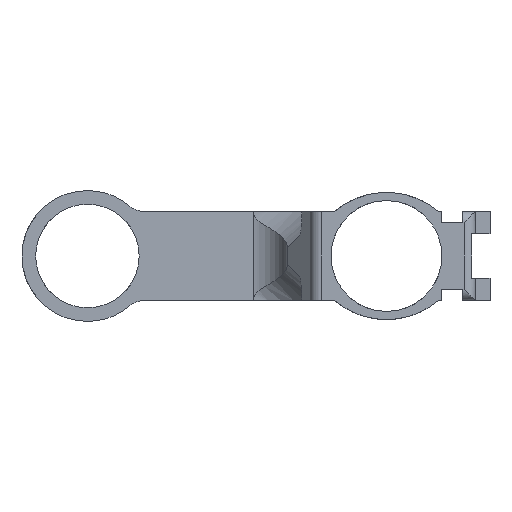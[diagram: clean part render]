
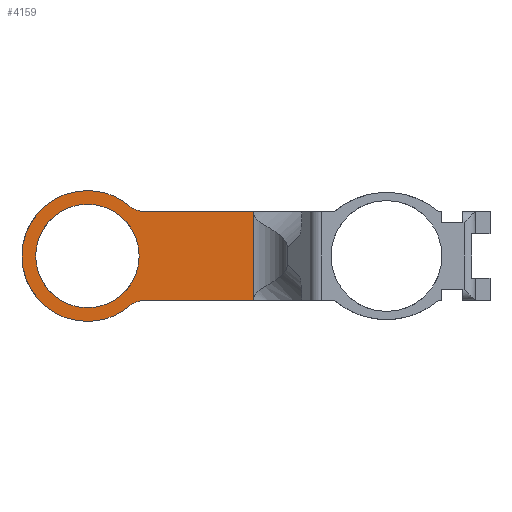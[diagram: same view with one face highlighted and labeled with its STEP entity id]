
A CAD part, left-side view. The second image highlights one B-rep face of the part: STEP entity #4159.
In plain terms, the highlighted planar face has unit normal (-1, 0, 0).
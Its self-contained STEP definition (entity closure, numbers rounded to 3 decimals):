
#380 = FACE_OUTER_BOUND ( 'NONE', #5228, .T. ) ;
#385 = FACE_BOUND ( 'NONE', #5230, .T. ) ;
#406 = CIRCLE ( 'NONE', #5538, 7. ) ;
#436 = CIRCLE ( 'NONE', #5544, 8.85 ) ;
#573 = LINE ( 'NONE', #3904, #576 ) ;
#576 = VECTOR ( 'NONE', #3905, 1000. ) ;
#577 = CIRCLE ( 'NONE', #3512, 8.85 ) ;
#1004 = CIRCLE ( 'NONE', #3519, 7. ) ;
#1006 = LINE ( 'NONE', #1348, #1010 ) ;
#1007 = LINE ( 'NONE', #1346, #1008 ) ;
#1008 = VECTOR ( 'NONE', #1347, 1000. ) ;
#1009 = CIRCLE ( 'NONE', #3520, 3. ) ;
#1010 = VECTOR ( 'NONE', #1349, 1000. ) ;
#1011 = CIRCLE ( 'NONE', #3521, 3. ) ;
#1012 = LINE ( 'NONE', #1350, #1014 ) ;
#1014 = VECTOR ( 'NONE', #1351, 1000. ) ;
#1143 = CIRCLE ( 'NONE', #3552, 8.85 ) ;
#1304 = CARTESIAN_POINT ( 'NONE',  ( -14., 40.45, 0. ) ) ;
#1305 = DIRECTION ( 'NONE',  ( -1., 0., 0. ) ) ;
#1306 = DIRECTION ( 'NONE',  ( 0., 1., 0. ) ) ;
#1346 = CARTESIAN_POINT ( 'NONE',  ( -14., 18.048, 6. ) ) ;
#1347 = DIRECTION ( 'NONE',  ( 0., 0., 1. ) ) ;
#1348 = CARTESIAN_POINT ( 'NONE',  ( -14., 18.024, 5.976 ) ) ;
#1349 = DIRECTION ( 'NONE',  ( 0., -0.707, 0.707 ) ) ;
#1350 = CARTESIAN_POINT ( 'NONE',  ( -14., 18.024, -5.976 ) ) ;
#1351 = DIRECTION ( 'NONE',  ( 0., 0.707, 0.707 ) ) ;
#1352 = CARTESIAN_POINT ( 'NONE',  ( -14., 32.741, 9. ) ) ;
#1353 = DIRECTION ( 'NONE',  ( 1., 0., 0. ) ) ;
#1354 = DIRECTION ( 'NONE',  ( 0., 1., 0. ) ) ;
#1355 = CARTESIAN_POINT ( 'NONE',  ( -14., 32.741, -9. ) ) ;
#1356 = DIRECTION ( 'NONE',  ( 1., 0., 0. ) ) ;
#1357 = DIRECTION ( 'NONE',  ( 0., 1., 0. ) ) ;
#1808 = CARTESIAN_POINT ( 'NONE',  ( -14., 40.45, 0. ) ) ;
#1809 = DIRECTION ( 'NONE',  ( -1., 0., 0. ) ) ;
#1810 = DIRECTION ( 'NONE',  ( 0., 1., 0. ) ) ;
#2225 = CARTESIAN_POINT ( 'NONE',  ( -14., 24.039, -6. ) ) ;
#2226 = DIRECTION ( 'NONE',  ( 0., -1., 0. ) ) ;
#2457 = LINE ( 'NONE', #2225, #2460 ) ;
#2460 = VECTOR ( 'NONE', #2226, 1000. ) ;
#2681 = CARTESIAN_POINT ( 'NONE',  ( -14., 49.3, -8.85 ) ) ;
#2686 = DIRECTION ( 'NONE',  ( 1., 0., 0. ) ) ;
#2688 = PLANE ( 'NONE',  #5525 ) ;
#2690 = DIRECTION ( 'NONE',  ( 0., 1., 0. ) ) ;
#2842 = CARTESIAN_POINT ( 'NONE',  ( -14., 40.45, 0. ) ) ;
#2843 = DIRECTION ( 'NONE',  ( -1., 0., 0. ) ) ;
#2844 = DIRECTION ( 'NONE',  ( 0., 1., 0. ) ) ;
#3123 = CARTESIAN_POINT ( 'NONE',  ( -14., 40.45, 0. ) ) ;
#3124 = DIRECTION ( 'NONE',  ( -1., 0., 0. ) ) ;
#3125 = DIRECTION ( 'NONE',  ( 0., 1., 0. ) ) ;
#3235 = CARTESIAN_POINT ( 'NONE',  ( -14., 34.693, -6.722 ) ) ;
#3236 = CARTESIAN_POINT ( 'NONE',  ( -14., 40.45, -7. ) ) ;
#3238 = CARTESIAN_POINT ( 'NONE',  ( -14., 40.45, 7. ) ) ;
#3260 = CARTESIAN_POINT ( 'NONE',  ( -14., 40.45, 8.85 ) ) ;
#3268 = CARTESIAN_POINT ( 'NONE',  ( -14., 40.45, -8.85 ) ) ;
#3290 = CARTESIAN_POINT ( 'NONE',  ( -14., 32.741, -6. ) ) ;
#3295 = CARTESIAN_POINT ( 'NONE',  ( -14., 18., -6. ) ) ;
#3388 = CARTESIAN_POINT ( 'NONE',  ( -14., 18., 6. ) ) ;
#3392 = CARTESIAN_POINT ( 'NONE',  ( -14., 32.741, 6. ) ) ;
#3394 = CARTESIAN_POINT ( 'NONE',  ( -14., 34.693, 6.722 ) ) ;
#3433 = CARTESIAN_POINT ( 'NONE',  ( -14., 18.048, 5.952 ) ) ;
#3435 = CARTESIAN_POINT ( 'NONE',  ( -14., 18.048, -5.952 ) ) ;
#3512 = AXIS2_PLACEMENT_3D ( 'NONE', #3916, #3917, #3918 ) ;
#3519 = AXIS2_PLACEMENT_3D ( 'NONE', #1304, #1305, #1306 ) ;
#3520 = AXIS2_PLACEMENT_3D ( 'NONE', #1352, #1353, #1354 ) ;
#3521 = AXIS2_PLACEMENT_3D ( 'NONE', #1355, #1356, #1357 ) ;
#3552 = AXIS2_PLACEMENT_3D ( 'NONE', #1808, #1809, #1810 ) ;
#3904 = CARTESIAN_POINT ( 'NONE',  ( -14., 12.842, 6. ) ) ;
#3905 = DIRECTION ( 'NONE',  ( 0., 1., 0. ) ) ;
#3916 = CARTESIAN_POINT ( 'NONE',  ( -14., 40.45, 0. ) ) ;
#3917 = DIRECTION ( 'NONE',  ( -1., 0., 0. ) ) ;
#3918 = DIRECTION ( 'NONE',  ( 0., 1., 0. ) ) ;
#4159 = ADVANCED_FACE ( 'NONE', ( #380, #385 ), #2688, .F. ) ;
#4178 = EDGE_CURVE ( 'NONE', #4330, #4332, #406, .T. ) ;
#4208 = EDGE_CURVE ( 'NONE', #4354, #4362, #436, .T. ) ;
#4329 = VERTEX_POINT ( 'NONE', #3235 ) ;
#4330 = VERTEX_POINT ( 'NONE', #3236 ) ;
#4332 = VERTEX_POINT ( 'NONE', #3238 ) ;
#4354 = VERTEX_POINT ( 'NONE', #3260 ) ;
#4362 = VERTEX_POINT ( 'NONE', #3268 ) ;
#4384 = VERTEX_POINT ( 'NONE', #3290 ) ;
#4389 = VERTEX_POINT ( 'NONE', #3295 ) ;
#4482 = VERTEX_POINT ( 'NONE', #3388 ) ;
#4486 = VERTEX_POINT ( 'NONE', #3392 ) ;
#4488 = VERTEX_POINT ( 'NONE', #3394 ) ;
#4527 = VERTEX_POINT ( 'NONE', #3433 ) ;
#4529 = VERTEX_POINT ( 'NONE', #3435 ) ;
#4886 = EDGE_CURVE ( 'NONE', #4482, #4486, #573, .T. ) ;
#4890 = EDGE_CURVE ( 'NONE', #4488, #4354, #577, .T. ) ;
#5005 = ORIENTED_EDGE ( 'NONE', *, *, #5252, .T. ) ;
#5006 = ORIENTED_EDGE ( 'NONE', *, *, #5253, .T. ) ;
#5007 = ORIENTED_EDGE ( 'NONE', *, *, #4886, .T. ) ;
#5008 = ORIENTED_EDGE ( 'NONE', *, *, #5254, .T. ) ;
#5009 = ORIENTED_EDGE ( 'NONE', *, *, #4890, .T. ) ;
#5010 = ORIENTED_EDGE ( 'NONE', *, *, #4208, .T. ) ;
#5011 = ORIENTED_EDGE ( 'NONE', *, *, #5361, .T. ) ;
#5012 = ORIENTED_EDGE ( 'NONE', *, *, #5255, .T. ) ;
#5013 = ORIENTED_EDGE ( 'NONE', *, *, #5453, .T. ) ;
#5014 = ORIENTED_EDGE ( 'NONE', *, *, #5256, .T. ) ;
#5015 = ORIENTED_EDGE ( 'NONE', *, *, #4178, .F. ) ;
#5016 = ORIENTED_EDGE ( 'NONE', *, *, #5250, .F. ) ;
#5228 = EDGE_LOOP ( 'NONE', ( #5005, #5006, #5007, #5008, #5009, #5010, #5011, #5012, #5013, #5014 ) ) ;
#5230 = EDGE_LOOP ( 'NONE', ( #5015, #5016 ) ) ;
#5250 = EDGE_CURVE ( 'NONE', #4332, #4330, #1004, .T. ) ;
#5252 = EDGE_CURVE ( 'NONE', #4529, #4527, #1007, .T. ) ;
#5253 = EDGE_CURVE ( 'NONE', #4527, #4482, #1006, .T. ) ;
#5254 = EDGE_CURVE ( 'NONE', #4486, #4488, #1009, .T. ) ;
#5255 = EDGE_CURVE ( 'NONE', #4329, #4384, #1011, .T. ) ;
#5256 = EDGE_CURVE ( 'NONE', #4389, #4529, #1012, .T. ) ;
#5361 = EDGE_CURVE ( 'NONE', #4362, #4329, #1143, .T. ) ;
#5453 = EDGE_CURVE ( 'NONE', #4384, #4389, #2457, .T. ) ;
#5525 = AXIS2_PLACEMENT_3D ( 'NONE', #2681, #2686, #2690 ) ;
#5538 = AXIS2_PLACEMENT_3D ( 'NONE', #2842, #2843, #2844 ) ;
#5544 = AXIS2_PLACEMENT_3D ( 'NONE', #3123, #3124, #3125 ) ;
